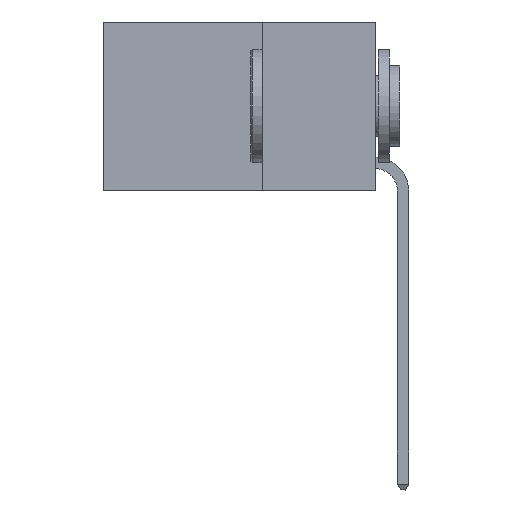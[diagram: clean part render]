
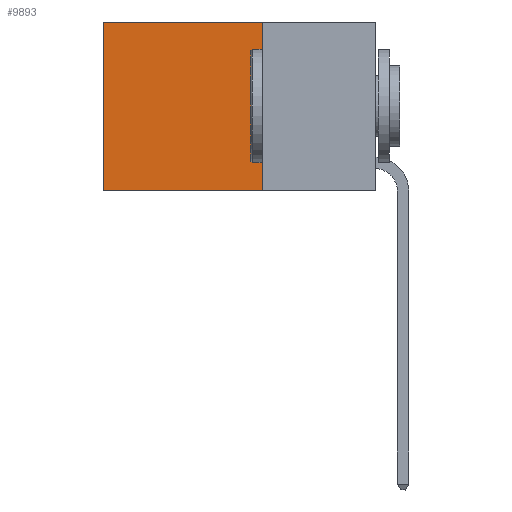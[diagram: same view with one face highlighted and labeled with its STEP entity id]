
A CAD part, left-side view. The second image highlights one B-rep face of the part: STEP entity #9893.
In plain terms, the highlighted planar face has unit normal (-1, 0, 0).
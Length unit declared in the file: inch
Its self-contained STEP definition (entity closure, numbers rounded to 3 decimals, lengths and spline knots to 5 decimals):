
#1045 = DIRECTION ( 'NONE',  ( 0., 0., -1. ) ) ;
#1205 = EDGE_CURVE ( 'NONE', #3146, #14385, #1980, .T. ) ;
#1980 = LINE ( 'NONE', #15913, #12004 ) ;
#2615 = CARTESIAN_POINT ( 'NONE',  ( 0.2625, 0.25, -0.37 ) ) ;
#2685 = CARTESIAN_POINT ( 'NONE',  ( 0.2625, 0.25, -0.37 ) ) ;
#3146 = VERTEX_POINT ( 'NONE', #11827 ) ;
#5325 = DIRECTION ( 'NONE',  ( 0., 0., -1. ) ) ;
#6386 = EDGE_LOOP ( 'NONE', ( #16363, #8932, #8237, #20329 ) ) ;
#6485 = VECTOR ( 'NONE', #5325, 39.37008 ) ;
#6659 = PLANE ( 'NONE',  #11630 ) ;
#7270 = LINE ( 'NONE', #2615, #16725 ) ;
#7883 = LINE ( 'NONE', #16242, #17349 ) ;
#8105 = VERTEX_POINT ( 'NONE', #2685 ) ;
#8233 = LINE ( 'NONE', #14715, #6485 ) ;
#8237 = ORIENTED_EDGE ( 'NONE', *, *, #23179, .F. ) ;
#8932 = ORIENTED_EDGE ( 'NONE', *, *, #23601, .F. ) ;
#9052 = VERTEX_POINT ( 'NONE', #9113 ) ;
#9113 = CARTESIAN_POINT ( 'NONE',  ( 0.2625, 0.6, -0.37 ) ) ;
#9893 = ADVANCED_FACE ( 'NONE', ( #16933 ), #6659, .F. ) ;
#11630 = AXIS2_PLACEMENT_3D ( 'NONE', #17942, #12328, #1045 ) ;
#11827 = CARTESIAN_POINT ( 'NONE',  ( 0.2625, 0.25, 0. ) ) ;
#12004 = VECTOR ( 'NONE', #16179, 39.37008 ) ;
#12328 = DIRECTION ( 'NONE',  ( 1., 0., 0. ) ) ;
#13881 = DIRECTION ( 'NONE',  ( 0., 1., 0. ) ) ;
#14385 = VERTEX_POINT ( 'NONE', #18193 ) ;
#14715 = CARTESIAN_POINT ( 'NONE',  ( 0.2625, 0.6, 0. ) ) ;
#15913 = CARTESIAN_POINT ( 'NONE',  ( 0.2625, 0.25, 0. ) ) ;
#16179 = DIRECTION ( 'NONE',  ( 0., 1., 0. ) ) ;
#16242 = CARTESIAN_POINT ( 'NONE',  ( 0.2625, 0.25, 0. ) ) ;
#16363 = ORIENTED_EDGE ( 'NONE', *, *, #17378, .T. ) ;
#16725 = VECTOR ( 'NONE', #13881, 39.37008 ) ;
#16933 = FACE_OUTER_BOUND ( 'NONE', #6386, .T. ) ;
#17349 = VECTOR ( 'NONE', #22012, 39.37008 ) ;
#17378 = EDGE_CURVE ( 'NONE', #14385, #9052, #8233, .T. ) ;
#17942 = CARTESIAN_POINT ( 'NONE',  ( 0.2625, 0.25, 0. ) ) ;
#18193 = CARTESIAN_POINT ( 'NONE',  ( 0.2625, 0.6, 0. ) ) ;
#20329 = ORIENTED_EDGE ( 'NONE', *, *, #1205, .T. ) ;
#22012 = DIRECTION ( 'NONE',  ( 0., 0., -1. ) ) ;
#23179 = EDGE_CURVE ( 'NONE', #3146, #8105, #7883, .T. ) ;
#23601 = EDGE_CURVE ( 'NONE', #8105, #9052, #7270, .T. ) ;
